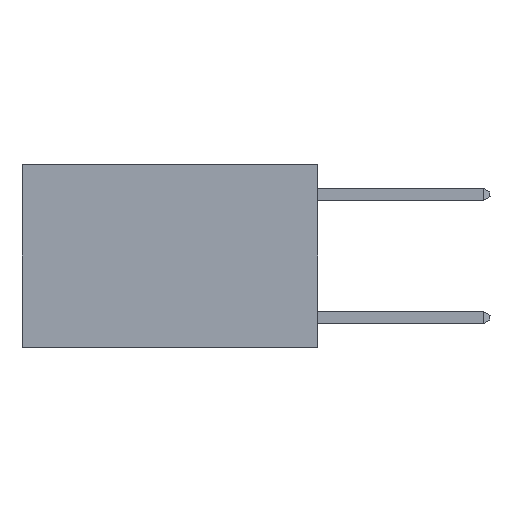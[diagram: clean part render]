
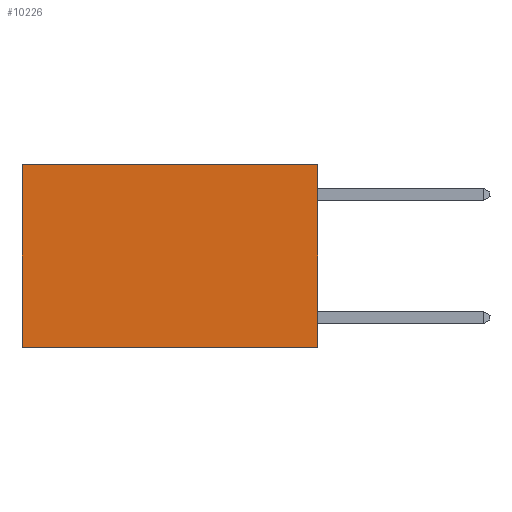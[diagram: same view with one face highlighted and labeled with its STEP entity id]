
A CAD part, left-side view. The second image highlights one B-rep face of the part: STEP entity #10226.
In plain terms, the highlighted planar face has unit normal (-1, 0, 0).
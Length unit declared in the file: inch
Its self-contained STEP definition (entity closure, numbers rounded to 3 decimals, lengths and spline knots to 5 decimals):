
#1778 = ORIENTED_EDGE ( 'NONE', *, *, #2700, .F. ) ;
#1855 = PLANE ( 'NONE',  #5361 ) ;
#1990 = CARTESIAN_POINT ( 'NONE',  ( 0.2625, 0., 0. ) ) ;
#2451 = LINE ( 'NONE', #1990, #15026 ) ;
#2614 = CARTESIAN_POINT ( 'NONE',  ( 0.2625, 0.6, 0. ) ) ;
#2700 = EDGE_CURVE ( 'NONE', #8890, #11850, #11837, .T. ) ;
#3653 = CARTESIAN_POINT ( 'NONE',  ( 0.2625, 0., 0. ) ) ;
#3816 = DIRECTION ( 'NONE',  ( 0., 0., -1. ) ) ;
#4205 = EDGE_LOOP ( 'NONE', ( #15087, #1778, #14257, #7198 ) ) ;
#5080 = FACE_OUTER_BOUND ( 'NONE', #4205, .T. ) ;
#5361 = AXIS2_PLACEMENT_3D ( 'NONE', #15479, #5802, #12907 ) ;
#5802 = DIRECTION ( 'NONE',  ( 1., 0., 0. ) ) ;
#5998 = DIRECTION ( 'NONE',  ( 0., 1., 0. ) ) ;
#6176 = CARTESIAN_POINT ( 'NONE',  ( 0.2625, 0.6, -0.37 ) ) ;
#6267 = VECTOR ( 'NONE', #5998, 39.37008 ) ;
#7198 = ORIENTED_EDGE ( 'NONE', *, *, #13694, .T. ) ;
#7318 = DIRECTION ( 'NONE',  ( 0., 1., 0. ) ) ;
#8736 = LINE ( 'NONE', #3653, #6267 ) ;
#8890 = VERTEX_POINT ( 'NONE', #10506 ) ;
#9712 = EDGE_CURVE ( 'NONE', #12507, #8890, #2451, .T. ) ;
#10226 = ADVANCED_FACE ( 'NONE', ( #5080 ), #1855, .F. ) ;
#10506 = CARTESIAN_POINT ( 'NONE',  ( 0.2625, 0., -0.37 ) ) ;
#10740 = LINE ( 'NONE', #2614, #12647 ) ;
#10783 = CARTESIAN_POINT ( 'NONE',  ( 0.2625, 0., 0. ) ) ;
#11082 = VECTOR ( 'NONE', #7318, 39.37008 ) ;
#11837 = LINE ( 'NONE', #15446, #11082 ) ;
#11850 = VERTEX_POINT ( 'NONE', #6176 ) ;
#12040 = EDGE_CURVE ( 'NONE', #15726, #11850, #10740, .T. ) ;
#12507 = VERTEX_POINT ( 'NONE', #10783 ) ;
#12647 = VECTOR ( 'NONE', #13752, 39.37008 ) ;
#12907 = DIRECTION ( 'NONE',  ( 0., 0., -1. ) ) ;
#13694 = EDGE_CURVE ( 'NONE', #12507, #15726, #8736, .T. ) ;
#13752 = DIRECTION ( 'NONE',  ( 0., 0., -1. ) ) ;
#14257 = ORIENTED_EDGE ( 'NONE', *, *, #9712, .F. ) ;
#15026 = VECTOR ( 'NONE', #3816, 39.37008 ) ;
#15087 = ORIENTED_EDGE ( 'NONE', *, *, #12040, .T. ) ;
#15446 = CARTESIAN_POINT ( 'NONE',  ( 0.2625, 0., -0.37 ) ) ;
#15479 = CARTESIAN_POINT ( 'NONE',  ( 0.2625, 0., 0. ) ) ;
#15538 = CARTESIAN_POINT ( 'NONE',  ( 0.2625, 0.6, 0. ) ) ;
#15726 = VERTEX_POINT ( 'NONE', #15538 ) ;
